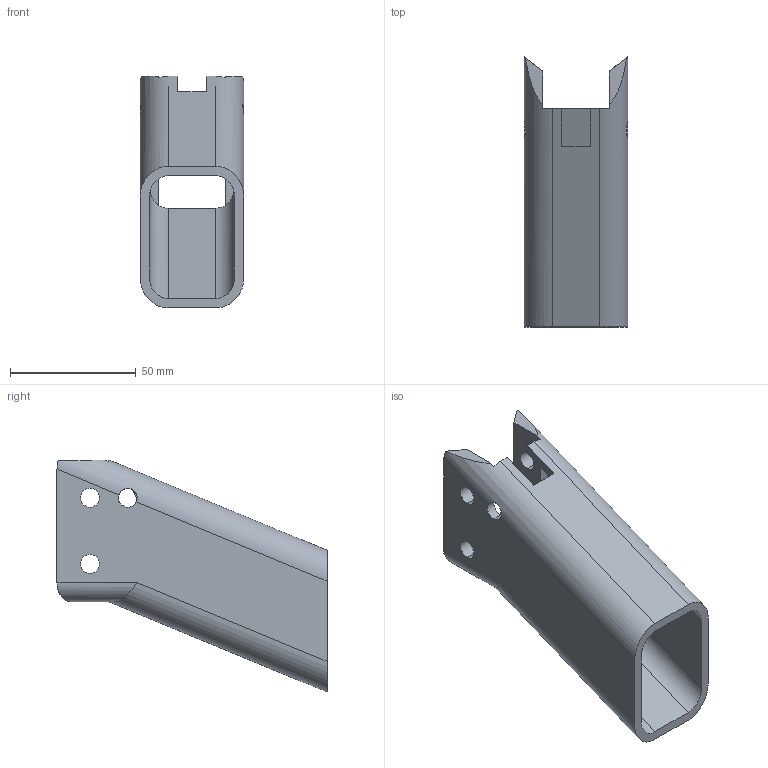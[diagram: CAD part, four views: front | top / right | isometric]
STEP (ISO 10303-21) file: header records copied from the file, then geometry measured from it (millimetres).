
FILE_DESCRIPTION (( 'STEP AP203' ), '1' );
FILE_NAME ('Grip.STEP', '2013-09-22T12:21:44', ( '' ), ( '' ), 'SwSTEP 2.0', 'SolidWorks 2013', '' );
FILE_SCHEMA (( 'CONFIG_CONTROL_DESIGN' ));
Length unit declared in the file: millimetre
Products named in the file (1): Grip
Bounding box: 41.25 x 107.24 x 92.13 mm (x, y, z)
Volume: 63457.9 mm3; surface area: 35995.3 mm2
Topology: 1 solids, 1 shells, 49 faces, 148 edges, 96 vertices
Faces by surface type: cylinder 24, plane 23, bspline 2
Entity records: 2389 total; most frequent: CARTESIAN_POINT 1030, ORIENTED_EDGE 296, DIRECTION 242, EDGE_CURVE 148, VERTEX_POINT 96, VECTOR 82, LINE 82, AXIS2_PLACEMENT_3D 80
